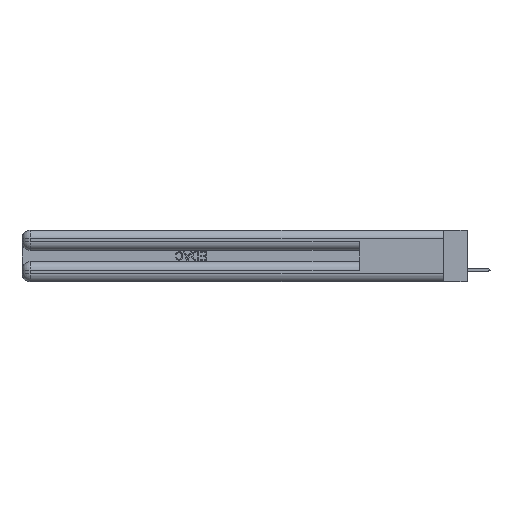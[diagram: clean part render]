
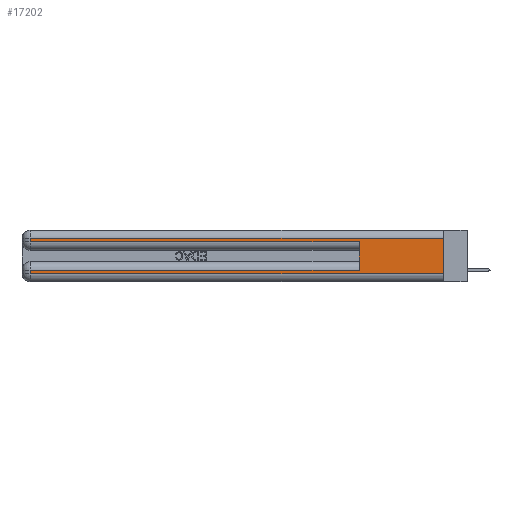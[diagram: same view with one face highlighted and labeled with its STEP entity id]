
A CAD part, left-side view. The second image highlights one B-rep face of the part: STEP entity #17202.
In plain terms, the highlighted planar face has unit normal (-1, 0, 0).
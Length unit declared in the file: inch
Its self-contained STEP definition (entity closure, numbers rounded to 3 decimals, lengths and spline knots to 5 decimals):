
#731 = VECTOR ( 'NONE', #38800, 39.37008 ) ;
#1205 = VERTEX_POINT ( 'NONE', #40135 ) ;
#1431 = EDGE_LOOP ( 'NONE', ( #5426, #51796, #51470, #6288, #30836, #17482, #51410, #32503 ) ) ;
#1677 = VERTEX_POINT ( 'NONE', #11873 ) ;
#2360 = CARTESIAN_POINT ( 'NONE',  ( 0., 0.6, 0.145 ) ) ;
#3786 = EDGE_CURVE ( 'NONE', #21435, #1677, #44036, .T. ) ;
#4118 = VERTEX_POINT ( 'NONE', #31924 ) ;
#4166 = EDGE_CURVE ( 'NONE', #21435, #4118, #16547, .T. ) ;
#5426 = ORIENTED_EDGE ( 'NONE', *, *, #34018, .F. ) ;
#5844 = EDGE_CURVE ( 'NONE', #1677, #43665, #24926, .T. ) ;
#6288 = ORIENTED_EDGE ( 'NONE', *, *, #26379, .T. ) ;
#8214 = VECTOR ( 'NONE', #34151, 39.37008 ) ;
#9171 = VECTOR ( 'NONE', #32502, 39.37008 ) ;
#9201 = CARTESIAN_POINT ( 'NONE',  ( 0., 2.94, 0.285 ) ) ;
#10448 = DIRECTION ( 'NONE',  ( 0., 1., 0. ) ) ;
#11738 = EDGE_CURVE ( 'NONE', #43665, #1205, #21845, .T. ) ;
#11873 = CARTESIAN_POINT ( 'NONE',  ( 0., 2.94, 0.085 ) ) ;
#13681 = AXIS2_PLACEMENT_3D ( 'NONE', #53577, #53389, #52352 ) ;
#14033 = LINE ( 'NONE', #17369, #8214 ) ;
#14285 = CARTESIAN_POINT ( 'NONE',  ( 0., 0., 0.285 ) ) ;
#16509 = FACE_OUTER_BOUND ( 'NONE', #1431, .T. ) ;
#16547 = LINE ( 'NONE', #2360, #9171 ) ;
#17202 = ADVANCED_FACE ( 'NONE', ( #16509 ), #20605, .F. ) ;
#17369 = CARTESIAN_POINT ( 'NONE',  ( 0., 2.94, 0.37 ) ) ;
#17482 = ORIENTED_EDGE ( 'NONE', *, *, #3786, .T. ) ;
#20605 = PLANE ( 'NONE',  #13681 ) ;
#21435 = VERTEX_POINT ( 'NONE', #42901 ) ;
#21845 = LINE ( 'NONE', #51269, #731 ) ;
#22529 = DIRECTION ( 'NONE',  ( 0., 0., -1. ) ) ;
#23738 = LINE ( 'NONE', #37261, #52434 ) ;
#24926 = LINE ( 'NONE', #43897, #49162 ) ;
#25159 = VECTOR ( 'NONE', #35301, 39.37008 ) ;
#26379 = EDGE_CURVE ( 'NONE', #40307, #4118, #29657, .T. ) ;
#28323 = LINE ( 'NONE', #35521, #34087 ) ;
#29421 = VERTEX_POINT ( 'NONE', #43178 ) ;
#29657 = LINE ( 'NONE', #14285, #25159 ) ;
#30836 = ORIENTED_EDGE ( 'NONE', *, *, #4166, .F. ) ;
#31562 = CARTESIAN_POINT ( 'NONE',  ( 0., 0., 0.31 ) ) ;
#31924 = CARTESIAN_POINT ( 'NONE',  ( 0., 0.6, 0.285 ) ) ;
#32502 = DIRECTION ( 'NONE',  ( 0., 0., 1. ) ) ;
#32503 = ORIENTED_EDGE ( 'NONE', *, *, #11738, .T. ) ;
#34018 = EDGE_CURVE ( 'NONE', #35333, #1205, #23738, .T. ) ;
#34087 = VECTOR ( 'NONE', #34777, 39.37008 ) ;
#34151 = DIRECTION ( 'NONE',  ( 0., 0., -1. ) ) ;
#34229 = EDGE_CURVE ( 'NONE', #35333, #29421, #28323, .T. ) ;
#34777 = DIRECTION ( 'NONE',  ( 0., 1., 0. ) ) ;
#35301 = DIRECTION ( 'NONE',  ( 0., -1., 0. ) ) ;
#35333 = VERTEX_POINT ( 'NONE', #31562 ) ;
#35521 = CARTESIAN_POINT ( 'NONE',  ( 0., 0., 0.31 ) ) ;
#37261 = CARTESIAN_POINT ( 'NONE',  ( 0., 0., 0.37 ) ) ;
#38800 = DIRECTION ( 'NONE',  ( 0., -1., 0. ) ) ;
#39963 = CARTESIAN_POINT ( 'NONE',  ( 0., 0., 0.085 ) ) ;
#40135 = CARTESIAN_POINT ( 'NONE',  ( 0., 0., 0.06 ) ) ;
#40307 = VERTEX_POINT ( 'NONE', #9201 ) ;
#42901 = CARTESIAN_POINT ( 'NONE',  ( 0., 0.6, 0.085 ) ) ;
#43178 = CARTESIAN_POINT ( 'NONE',  ( 0., 2.94, 0.31 ) ) ;
#43244 = EDGE_CURVE ( 'NONE', #29421, #40307, #14033, .T. ) ;
#43665 = VERTEX_POINT ( 'NONE', #49793 ) ;
#43897 = CARTESIAN_POINT ( 'NONE',  ( 0., 2.94, 0.37 ) ) ;
#44036 = LINE ( 'NONE', #39963, #47255 ) ;
#44502 = DIRECTION ( 'NONE',  ( 0., 0., -1. ) ) ;
#47255 = VECTOR ( 'NONE', #10448, 39.37008 ) ;
#49162 = VECTOR ( 'NONE', #44502, 39.37008 ) ;
#49793 = CARTESIAN_POINT ( 'NONE',  ( 0., 2.94, 0.06 ) ) ;
#51269 = CARTESIAN_POINT ( 'NONE',  ( 0., 0., 0.06 ) ) ;
#51410 = ORIENTED_EDGE ( 'NONE', *, *, #5844, .T. ) ;
#51470 = ORIENTED_EDGE ( 'NONE', *, *, #43244, .T. ) ;
#51796 = ORIENTED_EDGE ( 'NONE', *, *, #34229, .T. ) ;
#52352 = DIRECTION ( 'NONE',  ( 0., 0., -1. ) ) ;
#52434 = VECTOR ( 'NONE', #22529, 39.37008 ) ;
#53389 = DIRECTION ( 'NONE',  ( 1., 0., 0. ) ) ;
#53577 = CARTESIAN_POINT ( 'NONE',  ( 0., 0., 0.37 ) ) ;
